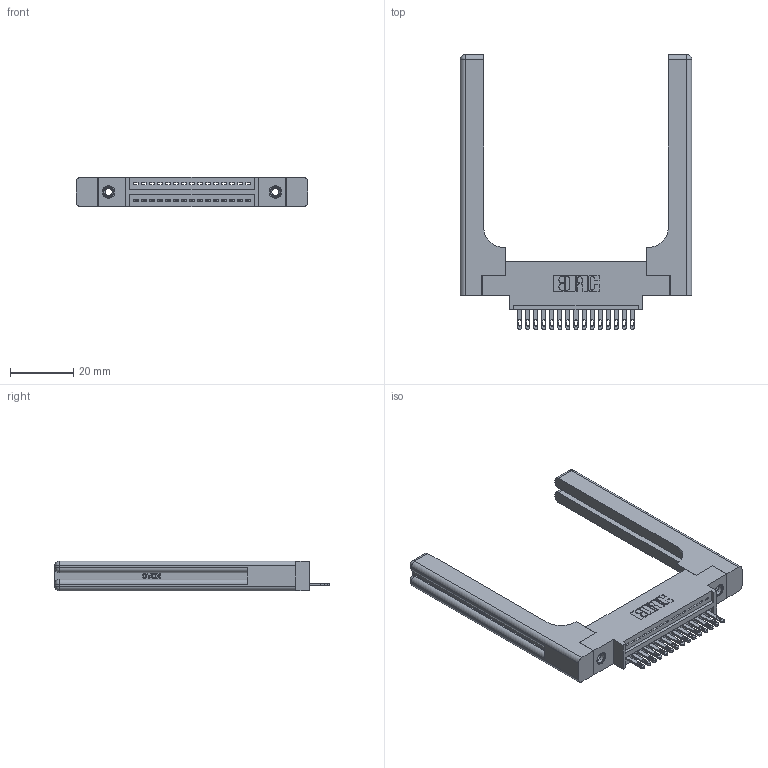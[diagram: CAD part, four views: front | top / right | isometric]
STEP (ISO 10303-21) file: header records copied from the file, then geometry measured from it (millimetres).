
FILE_DESCRIPTION (( 'STEP AP203' ), '1' );
FILE_NAME ('345-015-500-658.STEP', '2019-10-04T11:37:08', ( '' ), ( '' ), 'SwSTEP 2.0', 'SolidWorks 2016', '' );
FILE_SCHEMA (( 'CONFIG_CONTROL_DESIGN' ));
Length unit declared in the file: inch
Products named in the file (5): 345 Part_0.170 Offset - 0.156 Dia-TH; 345-015-500-658; 345-292-001_345-293-100; 345-220-058_345-220-058; 345-250-001_345-250-001-102
Assembly tree (20 placements, depth 2):
  345-015-500-658
    345 Part_0.170 Offset - 0.156 Dia-TH
    345-292-001_345-293-100  x15
    345-250-001_345-250-001-102  x2
    345-220-058_345-220-058  x2
Bounding box: 73.13 x 86.79 x 9.4 mm (x, y, z)
Volume: 15125.3 mm3; surface area: 13896.7 mm2
Topology: 20 solids, 20 shells, 1196 faces, 3539 edges, 2338 vertices
Faces by surface type: plane 742, cylinder 394, bspline 36, cone 12, sphere 8, torus 4
Entity records: 20168 total; most frequent: CARTESIAN_POINT 4466, ORIENTED_EDGE 3212, DIRECTION 2888, EDGE_CURVE 1606, LINE 1318, VECTOR 1318, VERTEX_POINT 1062, AXIS2_PLACEMENT_3D 785
